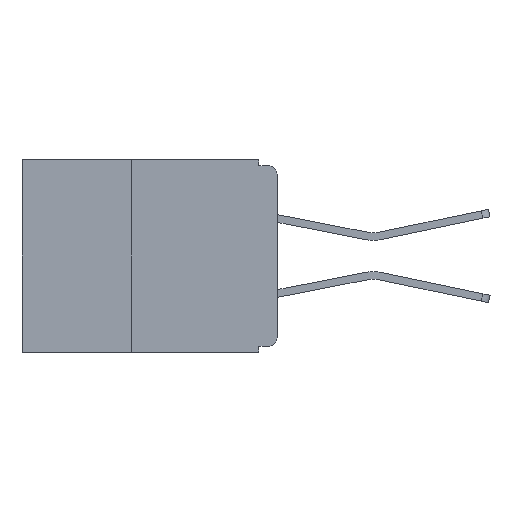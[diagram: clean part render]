
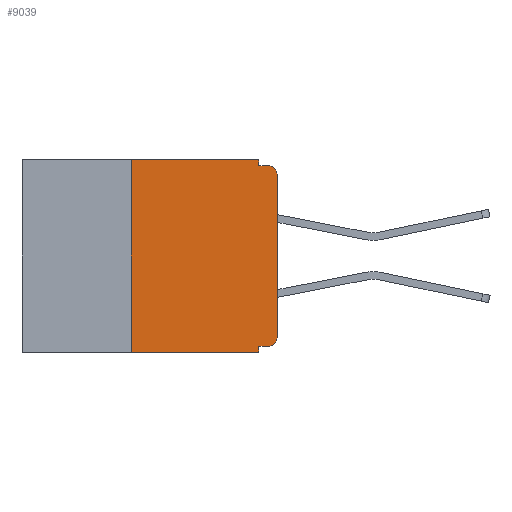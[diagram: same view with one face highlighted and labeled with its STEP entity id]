
A CAD part, left-side view. The second image highlights one B-rep face of the part: STEP entity #9039.
In plain terms, the highlighted planar face has unit normal (-1, 0, 0).
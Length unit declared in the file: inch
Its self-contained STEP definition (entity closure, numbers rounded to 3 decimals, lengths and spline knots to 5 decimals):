
#7 = DIRECTION ( 'NONE',  ( -1., 0., 0. ) ) ;
#256 = ORIENTED_EDGE ( 'NONE', *, *, #10077, .F. ) ;
#692 = EDGE_CURVE ( 'NONE', #11190, #14847, #7951, .T. ) ;
#745 = DIRECTION ( 'NONE',  ( -1., 0., 0. ) ) ;
#830 = ORIENTED_EDGE ( 'NONE', *, *, #3805, .T. ) ;
#846 = CARTESIAN_POINT ( 'NONE',  ( 0., 0.015, -0.32 ) ) ;
#856 = CARTESIAN_POINT ( 'NONE',  ( 0., 0.25, -0.33 ) ) ;
#921 = CARTESIAN_POINT ( 'NONE',  ( 0., 0.031, 0. ) ) ;
#968 = EDGE_CURVE ( 'NONE', #15236, #10081, #6324, .T. ) ;
#1276 = EDGE_CURVE ( 'NONE', #5455, #15236, #12896, .T. ) ;
#1854 = LINE ( 'NONE', #15828, #16825 ) ;
#1929 = DIRECTION ( 'NONE',  ( 0., -1., 0. ) ) ;
#2012 = VERTEX_POINT ( 'NONE', #12859 ) ;
#2090 = DIRECTION ( 'NONE',  ( 1., 0., 0. ) ) ;
#2218 = VERTEX_POINT ( 'NONE', #12836 ) ;
#2339 = VECTOR ( 'NONE', #12680, 39.37008 ) ;
#2424 = LINE ( 'NONE', #4210, #13525 ) ;
#2477 = VERTEX_POINT ( 'NONE', #16195 ) ;
#2699 = AXIS2_PLACEMENT_3D ( 'NONE', #9402, #745, #10856 ) ;
#2856 = AXIS2_PLACEMENT_3D ( 'NONE', #17289, #2090, #10092 ) ;
#3229 = LINE ( 'NONE', #12718, #2339 ) ;
#3350 = AXIS2_PLACEMENT_3D ( 'NONE', #16737, #7, #4773 ) ;
#3420 = DIRECTION ( 'NONE',  ( 0., 0., -1. ) ) ;
#3579 = CARTESIAN_POINT ( 'NONE',  ( 0., 0.031, -0.33 ) ) ;
#3793 = ORIENTED_EDGE ( 'NONE', *, *, #10766, .F. ) ;
#3805 = EDGE_CURVE ( 'NONE', #14847, #2477, #3229, .T. ) ;
#4210 = CARTESIAN_POINT ( 'NONE',  ( 0., 0.031, -0.33 ) ) ;
#4773 = DIRECTION ( 'NONE',  ( 0., 0., -1. ) ) ;
#5455 = VERTEX_POINT ( 'NONE', #12155 ) ;
#5568 = ORIENTED_EDGE ( 'NONE', *, *, #9923, .F. ) ;
#5616 = ORIENTED_EDGE ( 'NONE', *, *, #692, .T. ) ;
#5859 = LINE ( 'NONE', #14982, #8800 ) ;
#6324 = LINE ( 'NONE', #10774, #10173 ) ;
#7095 = DIRECTION ( 'NONE',  ( 0., -1., 0. ) ) ;
#7951 = CIRCLE ( 'NONE', #3350, 0.015 ) ;
#8123 = DIRECTION ( 'NONE',  ( 0., 1., 0. ) ) ;
#8189 = LINE ( 'NONE', #10638, #15939 ) ;
#8285 = ORIENTED_EDGE ( 'NONE', *, *, #968, .F. ) ;
#8332 = EDGE_CURVE ( 'NONE', #5455, #17095, #1854, .T. ) ;
#8658 = PLANE ( 'NONE',  #2856 ) ;
#8800 = VECTOR ( 'NONE', #1929, 39.37008 ) ;
#9039 = ADVANCED_FACE ( 'NONE', ( #12231 ), #8658, .F. ) ;
#9402 = CARTESIAN_POINT ( 'NONE',  ( 0., 0.015, -0.025 ) ) ;
#9903 = VERTEX_POINT ( 'NONE', #11927 ) ;
#9911 = VECTOR ( 'NONE', #8123, 39.37008 ) ;
#9923 = EDGE_CURVE ( 'NONE', #2218, #2012, #5859, .T. ) ;
#10077 = EDGE_CURVE ( 'NONE', #11190, #9903, #15646, .T. ) ;
#10081 = VERTEX_POINT ( 'NONE', #921 ) ;
#10092 = DIRECTION ( 'NONE',  ( 0., 0., -1. ) ) ;
#10173 = VECTOR ( 'NONE', #16871, 39.37008 ) ;
#10458 = CARTESIAN_POINT ( 'NONE',  ( 0., 0., -0.305 ) ) ;
#10638 = CARTESIAN_POINT ( 'NONE',  ( 0., 0.031, 0. ) ) ;
#10766 = EDGE_CURVE ( 'NONE', #9903, #17095, #2424, .T. ) ;
#10774 = CARTESIAN_POINT ( 'NONE',  ( 0., 0.437, 0. ) ) ;
#10856 = DIRECTION ( 'NONE',  ( 0., 0., -1. ) ) ;
#11190 = VERTEX_POINT ( 'NONE', #846 ) ;
#11292 = CARTESIAN_POINT ( 'NONE',  ( 0., 0.25, 0. ) ) ;
#11317 = EDGE_LOOP ( 'NONE', ( #830, #16409, #5568, #14227, #8285, #11963, #15998, #3793, #256, #5616 ) ) ;
#11330 = DIRECTION ( 'NONE',  ( 0., 0., 1. ) ) ;
#11927 = CARTESIAN_POINT ( 'NONE',  ( 0., 0.031, -0.32 ) ) ;
#11963 = ORIENTED_EDGE ( 'NONE', *, *, #1276, .F. ) ;
#12155 = CARTESIAN_POINT ( 'NONE',  ( 0., 0.25, -0.33 ) ) ;
#12231 = FACE_OUTER_BOUND ( 'NONE', #11317, .T. ) ;
#12441 = VECTOR ( 'NONE', #11330, 39.37008 ) ;
#12680 = DIRECTION ( 'NONE',  ( 0., 0., 1. ) ) ;
#12718 = CARTESIAN_POINT ( 'NONE',  ( 0., 0., 0. ) ) ;
#12836 = CARTESIAN_POINT ( 'NONE',  ( 0., 0.031, -0.01 ) ) ;
#12859 = CARTESIAN_POINT ( 'NONE',  ( 0., 0.015, -0.01 ) ) ;
#12863 = DIRECTION ( 'NONE',  ( 0., 0., -1. ) ) ;
#12896 = LINE ( 'NONE', #856, #12441 ) ;
#13525 = VECTOR ( 'NONE', #12863, 39.37008 ) ;
#14227 = ORIENTED_EDGE ( 'NONE', *, *, #17664, .F. ) ;
#14847 = VERTEX_POINT ( 'NONE', #10458 ) ;
#14982 = CARTESIAN_POINT ( 'NONE',  ( 0., 0., -0.01 ) ) ;
#14999 = EDGE_CURVE ( 'NONE', #2477, #2012, #15588, .T. ) ;
#15236 = VERTEX_POINT ( 'NONE', #11292 ) ;
#15365 = CARTESIAN_POINT ( 'NONE',  ( 0., 0., -0.32 ) ) ;
#15588 = CIRCLE ( 'NONE', #2699, 0.015 ) ;
#15646 = LINE ( 'NONE', #15365, #9911 ) ;
#15828 = CARTESIAN_POINT ( 'NONE',  ( 0., 0.437, -0.33 ) ) ;
#15939 = VECTOR ( 'NONE', #3420, 39.37008 ) ;
#15998 = ORIENTED_EDGE ( 'NONE', *, *, #8332, .T. ) ;
#16195 = CARTESIAN_POINT ( 'NONE',  ( 0., 0., -0.025 ) ) ;
#16409 = ORIENTED_EDGE ( 'NONE', *, *, #14999, .T. ) ;
#16737 = CARTESIAN_POINT ( 'NONE',  ( 0., 0.015, -0.305 ) ) ;
#16825 = VECTOR ( 'NONE', #7095, 39.37008 ) ;
#16871 = DIRECTION ( 'NONE',  ( 0., -1., 0. ) ) ;
#17095 = VERTEX_POINT ( 'NONE', #3579 ) ;
#17289 = CARTESIAN_POINT ( 'NONE',  ( 0., 0.437, 0. ) ) ;
#17664 = EDGE_CURVE ( 'NONE', #10081, #2218, #8189, .T. ) ;
